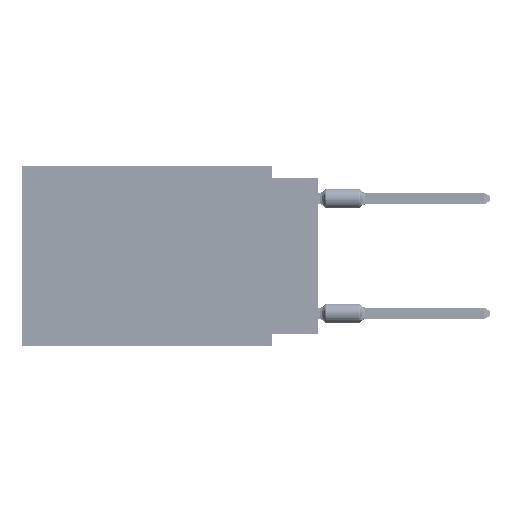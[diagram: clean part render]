
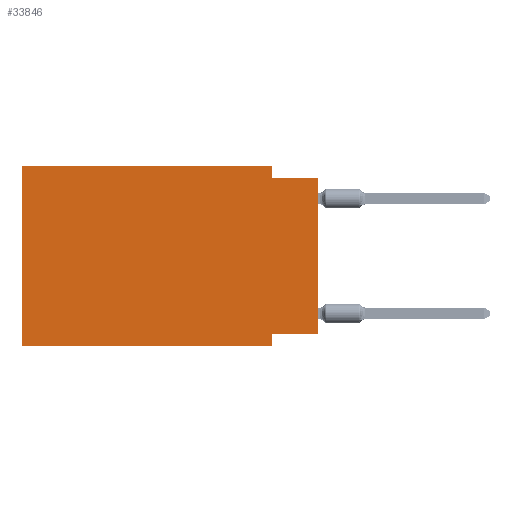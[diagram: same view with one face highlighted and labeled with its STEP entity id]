
A CAD part, left-side view. The second image highlights one B-rep face of the part: STEP entity #33846.
In plain terms, the highlighted planar face has unit normal (-1, 0, 0).
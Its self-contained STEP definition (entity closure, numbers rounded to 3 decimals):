
#212 = CARTESIAN_POINT ( 'NONE',  ( 0., 0., -9.271 ) ) ;
#2520 = LINE ( 'NONE', #72586, #16515 ) ;
#7403 = PLANE ( 'NONE',  #34169 ) ;
#9190 = VERTEX_POINT ( 'NONE', #28382 ) ;
#10363 = ORIENTED_EDGE ( 'NONE', *, *, #26351, .T. ) ;
#12016 = CARTESIAN_POINT ( 'NONE',  ( 0., 16.383, 0. ) ) ;
#13055 = DIRECTION ( 'NONE',  ( 0., 1., 0. ) ) ;
#14192 = ORIENTED_EDGE ( 'NONE', *, *, #51603, .F. ) ;
#14321 = LINE ( 'NONE', #212, #30690 ) ;
#15075 = DIRECTION ( 'NONE',  ( 0., 0., -1. ) ) ;
#16515 = VECTOR ( 'NONE', #27318, 1000. ) ;
#17342 = EDGE_CURVE ( 'NONE', #58026, #27510, #32186, .T. ) ;
#17831 = ORIENTED_EDGE ( 'NONE', *, *, #52171, .F. ) ;
#18192 = CARTESIAN_POINT ( 'NONE',  ( 0., 16.383, -9.906 ) ) ;
#20799 = CARTESIAN_POINT ( 'NONE',  ( 0., 2.54, -9.906 ) ) ;
#23473 = ORIENTED_EDGE ( 'NONE', *, *, #59229, .F. ) ;
#24663 = ORIENTED_EDGE ( 'NONE', *, *, #29417, .F. ) ;
#25766 = EDGE_LOOP ( 'NONE', ( #10363, #61966, #17831, #14192, #23473, #73926, #24663, #56263 ) ) ;
#25770 = DIRECTION ( 'NONE',  ( 0., -1., 0. ) ) ;
#26072 = CARTESIAN_POINT ( 'NONE',  ( 0., 2.54, -0.635 ) ) ;
#26351 = EDGE_CURVE ( 'NONE', #55538, #27510, #40972, .T. ) ;
#27318 = DIRECTION ( 'NONE',  ( 0., 0., -1. ) ) ;
#27510 = VERTEX_POINT ( 'NONE', #61510 ) ;
#27761 = CARTESIAN_POINT ( 'NONE',  ( 0., 0., 0. ) ) ;
#27945 = VECTOR ( 'NONE', #62245, 1000. ) ;
#28382 = CARTESIAN_POINT ( 'NONE',  ( 0., 16.383, -9.906 ) ) ;
#28962 = VECTOR ( 'NONE', #80791, 1000. ) ;
#29417 = EDGE_CURVE ( 'NONE', #77268, #76503, #43495, .T. ) ;
#30346 = CARTESIAN_POINT ( 'NONE',  ( 0., 16.383, 0. ) ) ;
#30690 = VECTOR ( 'NONE', #13055, 1000. ) ;
#31354 = VERTEX_POINT ( 'NONE', #34831 ) ;
#31753 = CARTESIAN_POINT ( 'NONE',  ( 0., 0., -0.635 ) ) ;
#32186 = LINE ( 'NONE', #31753, #49143 ) ;
#33846 = ADVANCED_FACE ( 'NONE', ( #45846 ), #7403, .F. ) ;
#34169 = AXIS2_PLACEMENT_3D ( 'NONE', #59932, #79561, #15075 ) ;
#34831 = CARTESIAN_POINT ( 'NONE',  ( 0., 2.54, 0. ) ) ;
#38783 = CARTESIAN_POINT ( 'NONE',  ( 0., 2.54, -9.906 ) ) ;
#40972 = LINE ( 'NONE', #27761, #27945 ) ;
#43495 = LINE ( 'NONE', #38783, #62222 ) ;
#44763 = DIRECTION ( 'NONE',  ( 0., 0., -1. ) ) ;
#44882 = LINE ( 'NONE', #12016, #55350 ) ;
#45846 = FACE_OUTER_BOUND ( 'NONE', #25766, .T. ) ;
#49143 = VECTOR ( 'NONE', #25770, 1000. ) ;
#51077 = CARTESIAN_POINT ( 'NONE',  ( 0., 0., -9.271 ) ) ;
#51603 = EDGE_CURVE ( 'NONE', #51824, #31354, #79088, .T. ) ;
#51824 = VERTEX_POINT ( 'NONE', #30346 ) ;
#52171 = EDGE_CURVE ( 'NONE', #31354, #58026, #2520, .T. ) ;
#55350 = VECTOR ( 'NONE', #82910, 1000. ) ;
#55538 = VERTEX_POINT ( 'NONE', #51077 ) ;
#56263 = ORIENTED_EDGE ( 'NONE', *, *, #57129, .F. ) ;
#57129 = EDGE_CURVE ( 'NONE', #55538, #77268, #14321, .T. ) ;
#58026 = VERTEX_POINT ( 'NONE', #26072 ) ;
#59229 = EDGE_CURVE ( 'NONE', #9190, #51824, #44882, .T. ) ;
#59932 = CARTESIAN_POINT ( 'NONE',  ( 0., 16.383, 0. ) ) ;
#61510 = CARTESIAN_POINT ( 'NONE',  ( 0., 0., -0.635 ) ) ;
#61966 = ORIENTED_EDGE ( 'NONE', *, *, #17342, .F. ) ;
#62222 = VECTOR ( 'NONE', #44763, 1000. ) ;
#62245 = DIRECTION ( 'NONE',  ( 0., 0., 1. ) ) ;
#65483 = VECTOR ( 'NONE', #76269, 1000. ) ;
#67566 = CARTESIAN_POINT ( 'NONE',  ( 0., 16.383, 0. ) ) ;
#72586 = CARTESIAN_POINT ( 'NONE',  ( 0., 2.54, 0. ) ) ;
#73926 = ORIENTED_EDGE ( 'NONE', *, *, #79431, .T. ) ;
#76269 = DIRECTION ( 'NONE',  ( 0., -1., 0. ) ) ;
#76452 = CARTESIAN_POINT ( 'NONE',  ( 0., 2.54, -9.271 ) ) ;
#76503 = VERTEX_POINT ( 'NONE', #20799 ) ;
#77268 = VERTEX_POINT ( 'NONE', #76452 ) ;
#77955 = LINE ( 'NONE', #18192, #65483 ) ;
#79088 = LINE ( 'NONE', #67566, #28962 ) ;
#79431 = EDGE_CURVE ( 'NONE', #9190, #76503, #77955, .T. ) ;
#79561 = DIRECTION ( 'NONE',  ( 1., 0., 0. ) ) ;
#80791 = DIRECTION ( 'NONE',  ( 0., -1., 0. ) ) ;
#82910 = DIRECTION ( 'NONE',  ( 0., 0., 1. ) ) ;
